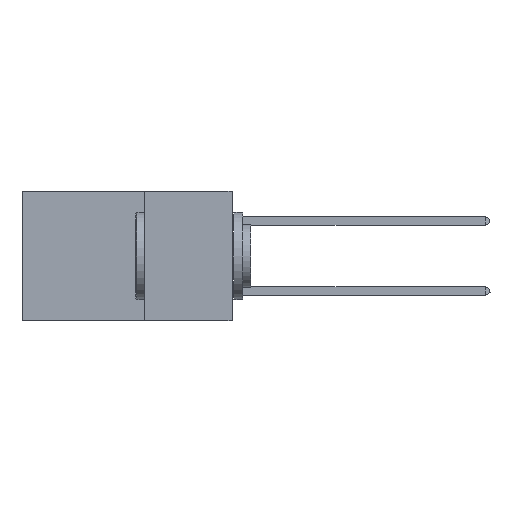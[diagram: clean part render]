
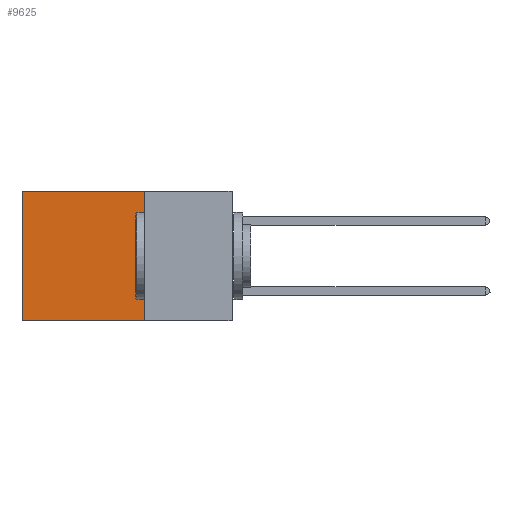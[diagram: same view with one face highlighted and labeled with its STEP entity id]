
A CAD part, left-side view. The second image highlights one B-rep face of the part: STEP entity #9625.
In plain terms, the highlighted planar face has unit normal (-1, 0, 0).
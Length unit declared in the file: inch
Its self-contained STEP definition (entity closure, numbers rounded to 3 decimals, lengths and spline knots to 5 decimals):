
#289 = PLANE ( 'NONE',  #15591 ) ;
#473 = CARTESIAN_POINT ( 'NONE',  ( 0.2875, 0.25, 0. ) ) ;
#696 = ORIENTED_EDGE ( 'NONE', *, *, #16938, .F. ) ;
#1589 = EDGE_CURVE ( 'NONE', #21508, #14666, #15334, .T. ) ;
#1922 = LINE ( 'NONE', #3352, #24180 ) ;
#2638 = DIRECTION ( 'NONE',  ( 0., 0., -1. ) ) ;
#2758 = DIRECTION ( 'NONE',  ( 1., 0., 0. ) ) ;
#3352 = CARTESIAN_POINT ( 'NONE',  ( 0.2875, 0.25, -0.37 ) ) ;
#3531 = LINE ( 'NONE', #473, #7581 ) ;
#4744 = VERTEX_POINT ( 'NONE', #14253 ) ;
#5698 = CARTESIAN_POINT ( 'NONE',  ( 0.2875, 0.25, 0. ) ) ;
#7581 = VECTOR ( 'NONE', #13689, 39.37008 ) ;
#7615 = EDGE_LOOP ( 'NONE', ( #13789, #696, #11807, #15658 ) ) ;
#8951 = CARTESIAN_POINT ( 'NONE',  ( 0.2875, 0.6, 0. ) ) ;
#9625 = ADVANCED_FACE ( 'NONE', ( #23546 ), #289, .F. ) ;
#10915 = CARTESIAN_POINT ( 'NONE',  ( 0.2875, 0.25, 0. ) ) ;
#11807 = ORIENTED_EDGE ( 'NONE', *, *, #1589, .F. ) ;
#12075 = CARTESIAN_POINT ( 'NONE',  ( 0.2875, 0.6, -0.37 ) ) ;
#13620 = DIRECTION ( 'NONE',  ( 0., 0., -1. ) ) ;
#13689 = DIRECTION ( 'NONE',  ( 0., 1., 0. ) ) ;
#13789 = ORIENTED_EDGE ( 'NONE', *, *, #21663, .T. ) ;
#14253 = CARTESIAN_POINT ( 'NONE',  ( 0.2875, 0.6, 0. ) ) ;
#14666 = VERTEX_POINT ( 'NONE', #32333 ) ;
#15334 = LINE ( 'NONE', #18781, #25014 ) ;
#15591 = AXIS2_PLACEMENT_3D ( 'NONE', #5698, #2758, #2638 ) ;
#15658 = ORIENTED_EDGE ( 'NONE', *, *, #16303, .T. ) ;
#15894 = LINE ( 'NONE', #8951, #21133 ) ;
#16303 = EDGE_CURVE ( 'NONE', #21508, #4744, #3531, .T. ) ;
#16938 = EDGE_CURVE ( 'NONE', #14666, #19786, #1922, .T. ) ;
#18781 = CARTESIAN_POINT ( 'NONE',  ( 0.2875, 0.25, 0. ) ) ;
#19786 = VERTEX_POINT ( 'NONE', #12075 ) ;
#21133 = VECTOR ( 'NONE', #22281, 39.37008 ) ;
#21508 = VERTEX_POINT ( 'NONE', #10915 ) ;
#21663 = EDGE_CURVE ( 'NONE', #4744, #19786, #15894, .T. ) ;
#22281 = DIRECTION ( 'NONE',  ( 0., 0., -1. ) ) ;
#23546 = FACE_OUTER_BOUND ( 'NONE', #7615, .T. ) ;
#24180 = VECTOR ( 'NONE', #31786, 39.37008 ) ;
#25014 = VECTOR ( 'NONE', #13620, 39.37008 ) ;
#31786 = DIRECTION ( 'NONE',  ( 0., 1., 0. ) ) ;
#32333 = CARTESIAN_POINT ( 'NONE',  ( 0.2875, 0.25, -0.37 ) ) ;
